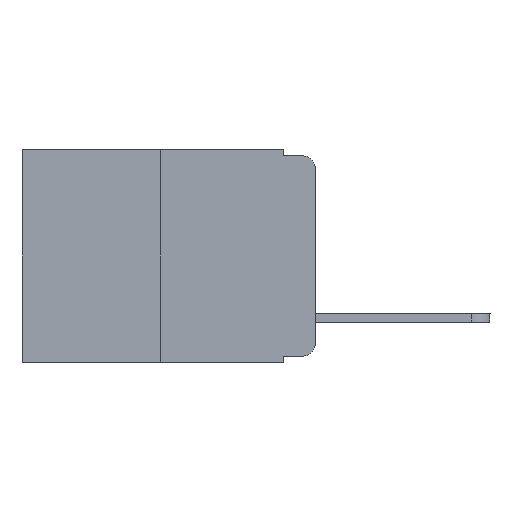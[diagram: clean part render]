
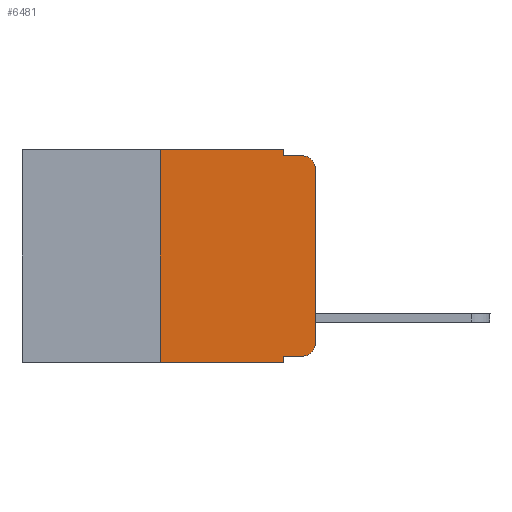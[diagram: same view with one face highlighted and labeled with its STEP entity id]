
A CAD part, left-side view. The second image highlights one B-rep face of the part: STEP entity #6481.
In plain terms, the highlighted planar face has unit normal (-1, 0, 0).
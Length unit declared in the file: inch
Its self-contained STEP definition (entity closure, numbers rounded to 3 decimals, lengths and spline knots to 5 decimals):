
#69 = VECTOR ( 'NONE', #3776, 39.37008 ) ;
#281 = EDGE_CURVE ( 'NONE', #11449, #11480, #4772, .T. ) ;
#323 = CARTESIAN_POINT ( 'NONE',  ( 0., 0.02, -0.313 ) ) ;
#411 = LINE ( 'NONE', #3490, #3545 ) ;
#628 = CARTESIAN_POINT ( 'NONE',  ( 0., 0.051, -0.333 ) ) ;
#703 = CARTESIAN_POINT ( 'NONE',  ( 0., 0.051, -0.333 ) ) ;
#993 = CARTESIAN_POINT ( 'NONE',  ( 0., 0.25, 0. ) ) ;
#1030 = AXIS2_PLACEMENT_3D ( 'NONE', #1130, #6335, #8514 ) ;
#1080 = CARTESIAN_POINT ( 'NONE',  ( 0., 0.25, -0.343 ) ) ;
#1095 = DIRECTION ( 'NONE',  ( 0., 0., -1. ) ) ;
#1130 = CARTESIAN_POINT ( 'NONE',  ( 0., 0.473, 0. ) ) ;
#1215 = EDGE_CURVE ( 'NONE', #7368, #11480, #10996, .T. ) ;
#1405 = DIRECTION ( 'NONE',  ( 0., -1., 0. ) ) ;
#1501 = ORIENTED_EDGE ( 'NONE', *, *, #10319, .T. ) ;
#1556 = LINE ( 'NONE', #8651, #12681 ) ;
#1819 = DIRECTION ( 'NONE',  ( 0., 0., -1. ) ) ;
#2026 = ORIENTED_EDGE ( 'NONE', *, *, #2153, .T. ) ;
#2153 = EDGE_CURVE ( 'NONE', #2200, #8759, #1556, .T. ) ;
#2200 = VERTEX_POINT ( 'NONE', #6235 ) ;
#2669 = EDGE_LOOP ( 'NONE', ( #2026, #11718, #4417, #10566, #7404, #7911, #8092, #3823, #1501, #6670 ) ) ;
#3087 = CARTESIAN_POINT ( 'NONE',  ( 0., 0., -0.03 ) ) ;
#3126 = VERTEX_POINT ( 'NONE', #993 ) ;
#3490 = CARTESIAN_POINT ( 'NONE',  ( 0., 0.25, 0. ) ) ;
#3545 = VECTOR ( 'NONE', #12247, 39.37008 ) ;
#3683 = DIRECTION ( 'NONE',  ( 0., -1., 0. ) ) ;
#3731 = VECTOR ( 'NONE', #10186, 39.37008 ) ;
#3776 = DIRECTION ( 'NONE',  ( 0., -1., 0. ) ) ;
#3823 = ORIENTED_EDGE ( 'NONE', *, *, #281, .F. ) ;
#4143 = AXIS2_PLACEMENT_3D ( 'NONE', #11683, #7387, #1095 ) ;
#4417 = ORIENTED_EDGE ( 'NONE', *, *, #7586, .F. ) ;
#4426 = VECTOR ( 'NONE', #1819, 39.37008 ) ;
#4772 = LINE ( 'NONE', #9312, #4426 ) ;
#4805 = FACE_OUTER_BOUND ( 'NONE', #2669, .T. ) ;
#4933 = CARTESIAN_POINT ( 'NONE',  ( 0., 0.051, 0. ) ) ;
#5282 = CARTESIAN_POINT ( 'NONE',  ( 0., 0.051, -0.343 ) ) ;
#5581 = VECTOR ( 'NONE', #1405, 39.37008 ) ;
#5942 = EDGE_CURVE ( 'NONE', #8759, #9342, #13295, .T. ) ;
#6235 = CARTESIAN_POINT ( 'NONE',  ( 0., 0., -0.313 ) ) ;
#6287 = CARTESIAN_POINT ( 'NONE',  ( 0., 0.02, -0.333 ) ) ;
#6307 = VERTEX_POINT ( 'NONE', #6287 ) ;
#6335 = DIRECTION ( 'NONE',  ( 1., 0., 0. ) ) ;
#6481 = ADVANCED_FACE ( 'NONE', ( #4805 ), #9595, .F. ) ;
#6670 = ORIENTED_EDGE ( 'NONE', *, *, #9289, .T. ) ;
#7368 = VERTEX_POINT ( 'NONE', #1080 ) ;
#7387 = DIRECTION ( 'NONE',  ( -1., 0., 0. ) ) ;
#7404 = ORIENTED_EDGE ( 'NONE', *, *, #12979, .F. ) ;
#7572 = DIRECTION ( 'NONE',  ( 0., 0., 1. ) ) ;
#7586 = EDGE_CURVE ( 'NONE', #9415, #9342, #12382, .T. ) ;
#7854 = CARTESIAN_POINT ( 'NONE',  ( 0., 0.473, 0. ) ) ;
#7894 = DIRECTION ( 'NONE',  ( -1., 0., 0. ) ) ;
#7911 = ORIENTED_EDGE ( 'NONE', *, *, #10212, .F. ) ;
#8092 = ORIENTED_EDGE ( 'NONE', *, *, #1215, .T. ) ;
#8514 = DIRECTION ( 'NONE',  ( 0., 0., -1. ) ) ;
#8643 = LINE ( 'NONE', #628, #69 ) ;
#8651 = CARTESIAN_POINT ( 'NONE',  ( 0., 0., 0. ) ) ;
#8759 = VERTEX_POINT ( 'NONE', #3087 ) ;
#8962 = DIRECTION ( 'NONE',  ( 0., 0., -1. ) ) ;
#9289 = EDGE_CURVE ( 'NONE', #6307, #2200, #10676, .T. ) ;
#9312 = CARTESIAN_POINT ( 'NONE',  ( 0., 0.051, 0. ) ) ;
#9342 = VERTEX_POINT ( 'NONE', #10991 ) ;
#9415 = VERTEX_POINT ( 'NONE', #13087 ) ;
#9595 = PLANE ( 'NONE',  #1030 ) ;
#9653 = VERTEX_POINT ( 'NONE', #13555 ) ;
#10186 = DIRECTION ( 'NONE',  ( 0., 0., -1. ) ) ;
#10212 = EDGE_CURVE ( 'NONE', #7368, #3126, #411, .T. ) ;
#10319 = EDGE_CURVE ( 'NONE', #11449, #6307, #8643, .T. ) ;
#10566 = ORIENTED_EDGE ( 'NONE', *, *, #12019, .F. ) ;
#10676 = CIRCLE ( 'NONE', #12226, 0.02 ) ;
#10991 = CARTESIAN_POINT ( 'NONE',  ( 0., 0.02, -0.01 ) ) ;
#10996 = LINE ( 'NONE', #11120, #11497 ) ;
#11120 = CARTESIAN_POINT ( 'NONE',  ( 0., 0.473, -0.343 ) ) ;
#11347 = LINE ( 'NONE', #7854, #5581 ) ;
#11449 = VERTEX_POINT ( 'NONE', #703 ) ;
#11480 = VERTEX_POINT ( 'NONE', #5282 ) ;
#11497 = VECTOR ( 'NONE', #3683, 39.37008 ) ;
#11683 = CARTESIAN_POINT ( 'NONE',  ( 0., 0.02, -0.03 ) ) ;
#11718 = ORIENTED_EDGE ( 'NONE', *, *, #5942, .T. ) ;
#12019 = EDGE_CURVE ( 'NONE', #9653, #9415, #12360, .T. ) ;
#12226 = AXIS2_PLACEMENT_3D ( 'NONE', #323, #7894, #8962 ) ;
#12247 = DIRECTION ( 'NONE',  ( 0., 0., 1. ) ) ;
#12360 = LINE ( 'NONE', #4933, #3731 ) ;
#12382 = LINE ( 'NONE', #13666, #13422 ) ;
#12681 = VECTOR ( 'NONE', #7572, 39.37008 ) ;
#12979 = EDGE_CURVE ( 'NONE', #3126, #9653, #11347, .T. ) ;
#13087 = CARTESIAN_POINT ( 'NONE',  ( 0., 0.051, -0.01 ) ) ;
#13295 = CIRCLE ( 'NONE', #4143, 0.02 ) ;
#13422 = VECTOR ( 'NONE', #13527, 39.37008 ) ;
#13527 = DIRECTION ( 'NONE',  ( 0., -1., 0. ) ) ;
#13555 = CARTESIAN_POINT ( 'NONE',  ( 0., 0.051, 0. ) ) ;
#13666 = CARTESIAN_POINT ( 'NONE',  ( 0., 0.051, -0.01 ) ) ;
